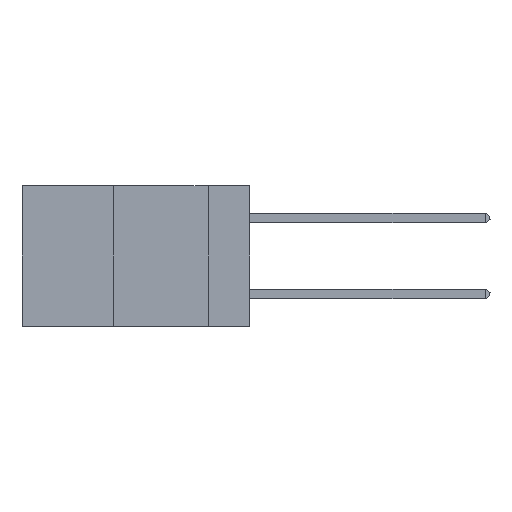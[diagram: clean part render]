
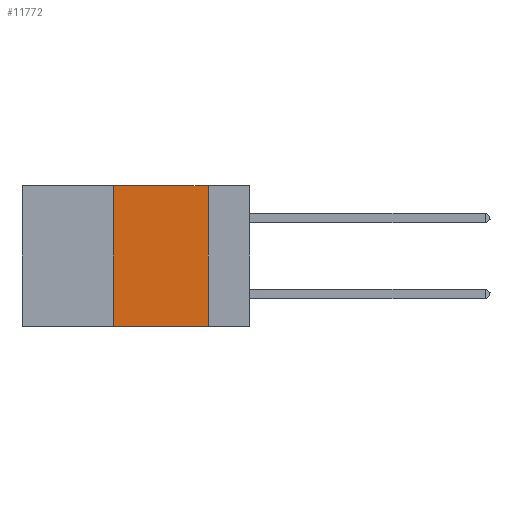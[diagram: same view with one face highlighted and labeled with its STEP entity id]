
A CAD part, left-side view. The second image highlights one B-rep face of the part: STEP entity #11772.
In plain terms, the highlighted planar face has unit normal (-1, 0, 0).
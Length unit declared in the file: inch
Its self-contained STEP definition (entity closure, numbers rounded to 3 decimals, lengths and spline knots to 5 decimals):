
#922 = VERTEX_POINT ( 'NONE', #35967 ) ;
#945 = AXIS2_PLACEMENT_3D ( 'NONE', #38042, #1972, #17059 ) ;
#1972 = DIRECTION ( 'NONE',  ( 1., 0., 0. ) ) ;
#2863 = ORIENTED_EDGE ( 'NONE', *, *, #4338, .T. ) ;
#4076 = EDGE_CURVE ( 'NONE', #23411, #23714, #13128, .T. ) ;
#4244 = EDGE_LOOP ( 'NONE', ( #33898, #36669, #35686, #2863 ) ) ;
#4338 = EDGE_CURVE ( 'NONE', #23411, #24397, #37652, .T. ) ;
#4729 = VECTOR ( 'NONE', #32409, 39.37008 ) ;
#7461 = CARTESIAN_POINT ( 'NONE',  ( 0., 0.36, 0. ) ) ;
#8974 = EDGE_CURVE ( 'NONE', #922, #24397, #11497, .T. ) ;
#10942 = CARTESIAN_POINT ( 'NONE',  ( 0., 0.11, -0.37 ) ) ;
#11394 = CARTESIAN_POINT ( 'NONE',  ( 0., 0.6, -0.37 ) ) ;
#11497 = LINE ( 'NONE', #32894, #18463 ) ;
#11772 = ADVANCED_FACE ( 'NONE', ( #35643 ), #34996, .F. ) ;
#13128 = LINE ( 'NONE', #24897, #27259 ) ;
#17059 = DIRECTION ( 'NONE',  ( 0., 0., -1. ) ) ;
#17280 = EDGE_CURVE ( 'NONE', #23714, #922, #36779, .T. ) ;
#17630 = CARTESIAN_POINT ( 'NONE',  ( 0., 0.36, -0.37 ) ) ;
#18463 = VECTOR ( 'NONE', #33019, 39.37008 ) ;
#23411 = VERTEX_POINT ( 'NONE', #17630 ) ;
#23714 = VERTEX_POINT ( 'NONE', #7461 ) ;
#24397 = VERTEX_POINT ( 'NONE', #10942 ) ;
#24897 = CARTESIAN_POINT ( 'NONE',  ( 0., 0.36, 0. ) ) ;
#27259 = VECTOR ( 'NONE', #33601, 39.37008 ) ;
#28758 = VECTOR ( 'NONE', #32509, 39.37008 ) ;
#29324 = CARTESIAN_POINT ( 'NONE',  ( 0., 0.6, 0. ) ) ;
#32409 = DIRECTION ( 'NONE',  ( 0., -1., 0. ) ) ;
#32509 = DIRECTION ( 'NONE',  ( 0., -1., 0. ) ) ;
#32894 = CARTESIAN_POINT ( 'NONE',  ( 0., 0.11, 0. ) ) ;
#33019 = DIRECTION ( 'NONE',  ( 0., 0., -1. ) ) ;
#33601 = DIRECTION ( 'NONE',  ( 0., 0., 1. ) ) ;
#33898 = ORIENTED_EDGE ( 'NONE', *, *, #8974, .F. ) ;
#34996 = PLANE ( 'NONE',  #945 ) ;
#35643 = FACE_OUTER_BOUND ( 'NONE', #4244, .T. ) ;
#35686 = ORIENTED_EDGE ( 'NONE', *, *, #4076, .F. ) ;
#35967 = CARTESIAN_POINT ( 'NONE',  ( 0., 0.11, 0. ) ) ;
#36669 = ORIENTED_EDGE ( 'NONE', *, *, #17280, .F. ) ;
#36779 = LINE ( 'NONE', #29324, #28758 ) ;
#37652 = LINE ( 'NONE', #11394, #4729 ) ;
#38042 = CARTESIAN_POINT ( 'NONE',  ( 0., 0.6, 0. ) ) ;
